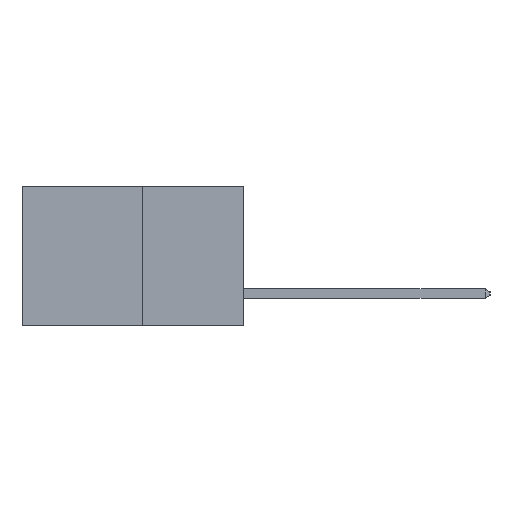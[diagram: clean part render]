
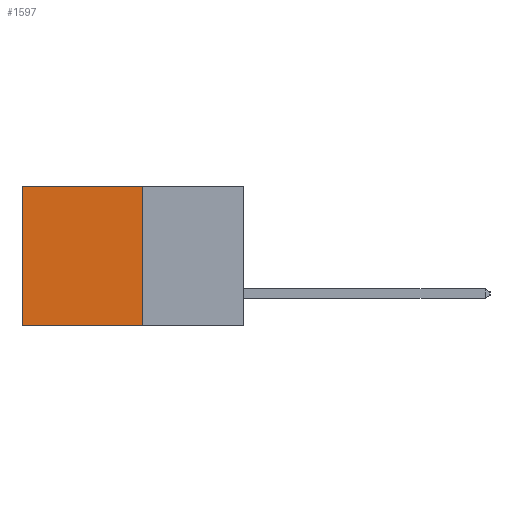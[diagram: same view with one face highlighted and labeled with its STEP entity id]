
A CAD part, left-side view. The second image highlights one B-rep face of the part: STEP entity #1597.
In plain terms, the highlighted planar face has unit normal (-1, 0, 0).
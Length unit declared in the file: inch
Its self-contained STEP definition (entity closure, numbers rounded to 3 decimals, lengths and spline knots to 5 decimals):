
#185 = LINE ( 'NONE', #1475, #511 ) ;
#475 = CARTESIAN_POINT ( 'NONE',  ( 0.277, 0.27, -0.37 ) ) ;
#511 = VECTOR ( 'NONE', #10492, 39.37008 ) ;
#1459 = EDGE_CURVE ( 'NONE', #10233, #7216, #185, .T. ) ;
#1475 = CARTESIAN_POINT ( 'NONE',  ( 0.277, 0.27, 0. ) ) ;
#1597 = ADVANCED_FACE ( 'NONE', ( #6975 ), #9443, .F. ) ;
#1783 = ORIENTED_EDGE ( 'NONE', *, *, #1459, .T. ) ;
#1870 = EDGE_CURVE ( 'NONE', #2871, #8962, #7228, .T. ) ;
#2856 = EDGE_LOOP ( 'NONE', ( #3811, #5992, #8134, #1783 ) ) ;
#2871 = VERTEX_POINT ( 'NONE', #475 ) ;
#3639 = CARTESIAN_POINT ( 'NONE',  ( 0.277, 0.27, -0.37 ) ) ;
#3811 = ORIENTED_EDGE ( 'NONE', *, *, #4021, .T. ) ;
#4021 = EDGE_CURVE ( 'NONE', #7216, #8962, #10528, .T. ) ;
#4242 = LINE ( 'NONE', #9854, #8268 ) ;
#4830 = AXIS2_PLACEMENT_3D ( 'NONE', #9421, #8974, #7043 ) ;
#5086 = VECTOR ( 'NONE', #8168, 39.37008 ) ;
#5868 = EDGE_CURVE ( 'NONE', #10233, #2871, #4242, .T. ) ;
#5928 = VECTOR ( 'NONE', #7388, 39.37008 ) ;
#5992 = ORIENTED_EDGE ( 'NONE', *, *, #1870, .F. ) ;
#6975 = FACE_OUTER_BOUND ( 'NONE', #2856, .T. ) ;
#7043 = DIRECTION ( 'NONE',  ( 0., 0., -1. ) ) ;
#7216 = VERTEX_POINT ( 'NONE', #9795 ) ;
#7228 = LINE ( 'NONE', #3639, #5086 ) ;
#7309 = CARTESIAN_POINT ( 'NONE',  ( 0.277, 0.59, -0.37 ) ) ;
#7388 = DIRECTION ( 'NONE',  ( 0., 0., -1. ) ) ;
#8134 = ORIENTED_EDGE ( 'NONE', *, *, #5868, .F. ) ;
#8168 = DIRECTION ( 'NONE',  ( 0., 1., 0. ) ) ;
#8268 = VECTOR ( 'NONE', #9022, 39.37008 ) ;
#8869 = CARTESIAN_POINT ( 'NONE',  ( 0.277, 0.59, -0.37 ) ) ;
#8962 = VERTEX_POINT ( 'NONE', #8869 ) ;
#8974 = DIRECTION ( 'NONE',  ( 1., 0., 0. ) ) ;
#9022 = DIRECTION ( 'NONE',  ( 0., 0., -1. ) ) ;
#9421 = CARTESIAN_POINT ( 'NONE',  ( 0.277, 0.27, -0.37 ) ) ;
#9443 = PLANE ( 'NONE',  #4830 ) ;
#9795 = CARTESIAN_POINT ( 'NONE',  ( 0.277, 0.59, 0. ) ) ;
#9854 = CARTESIAN_POINT ( 'NONE',  ( 0.277, 0.27, -0.37 ) ) ;
#10233 = VERTEX_POINT ( 'NONE', #10593 ) ;
#10492 = DIRECTION ( 'NONE',  ( 0., 1., 0. ) ) ;
#10528 = LINE ( 'NONE', #7309, #5928 ) ;
#10593 = CARTESIAN_POINT ( 'NONE',  ( 0.277, 0.27, 0. ) ) ;
